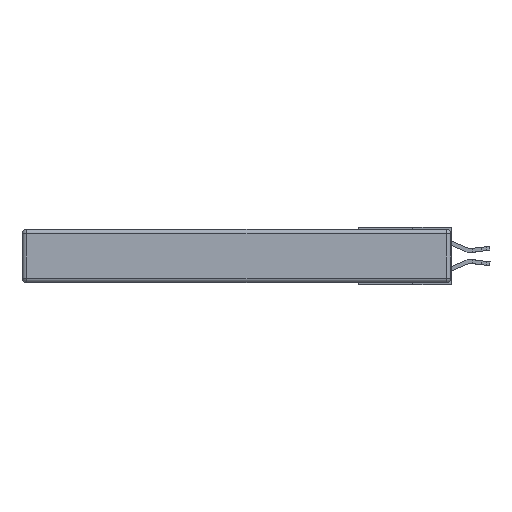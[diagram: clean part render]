
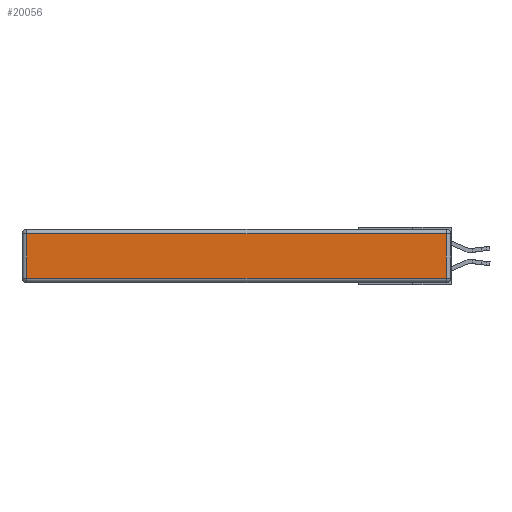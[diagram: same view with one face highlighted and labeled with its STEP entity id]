
A CAD part, left-side view. The second image highlights one B-rep face of the part: STEP entity #20056.
In plain terms, the highlighted planar face has unit normal (-1, 0, 0).
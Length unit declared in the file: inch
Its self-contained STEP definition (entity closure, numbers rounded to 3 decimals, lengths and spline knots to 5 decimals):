
#1045 = EDGE_CURVE ( 'NONE', #5660, #12351, #10678, .T. ) ;
#1574 = CARTESIAN_POINT ( 'NONE',  ( 0., 0., -0.313 ) ) ;
#1602 = CARTESIAN_POINT ( 'NONE',  ( 0., 0.03, -0.343 ) ) ;
#1655 = LINE ( 'NONE', #4994, #6934 ) ;
#3012 = LINE ( 'NONE', #17792, #17343 ) ;
#3937 = VERTEX_POINT ( 'NONE', #11427 ) ;
#4224 = VERTEX_POINT ( 'NONE', #5773 ) ;
#4994 = CARTESIAN_POINT ( 'NONE',  ( 0., 2.75, -0.03 ) ) ;
#5660 = VERTEX_POINT ( 'NONE', #11692 ) ;
#5773 = CARTESIAN_POINT ( 'NONE',  ( 0., 2.72, -0.313 ) ) ;
#5986 = DIRECTION ( 'NONE',  ( -1., 0., 0. ) ) ;
#6555 = AXIS2_PLACEMENT_3D ( 'NONE', #17345, #5986, #9339 ) ;
#6934 = VECTOR ( 'NONE', #19272, 39.37008 ) ;
#7466 = EDGE_CURVE ( 'NONE', #3937, #4224, #3012, .T. ) ;
#7895 = CARTESIAN_POINT ( 'NONE',  ( 0., 0.03, -0.03 ) ) ;
#9339 = DIRECTION ( 'NONE',  ( 0., 0., 1. ) ) ;
#9712 = ORIENTED_EDGE ( 'NONE', *, *, #1045, .T. ) ;
#9907 = VECTOR ( 'NONE', #17650, 39.37008 ) ;
#9934 = ORIENTED_EDGE ( 'NONE', *, *, #13434, .T. ) ;
#10027 = ORIENTED_EDGE ( 'NONE', *, *, #12484, .T. ) ;
#10678 = LINE ( 'NONE', #1602, #14408 ) ;
#11427 = CARTESIAN_POINT ( 'NONE',  ( 0., 2.72, -0.03 ) ) ;
#11692 = CARTESIAN_POINT ( 'NONE',  ( 0., 0.03, -0.313 ) ) ;
#12351 = VERTEX_POINT ( 'NONE', #7895 ) ;
#12484 = EDGE_CURVE ( 'NONE', #12351, #3937, #1655, .T. ) ;
#12853 = DIRECTION ( 'NONE',  ( 0., 0., 1. ) ) ;
#13434 = EDGE_CURVE ( 'NONE', #4224, #5660, #14176, .T. ) ;
#14115 = PLANE ( 'NONE',  #6555 ) ;
#14167 = EDGE_LOOP ( 'NONE', ( #9934, #9712, #10027, #20603 ) ) ;
#14176 = LINE ( 'NONE', #1574, #9907 ) ;
#14408 = VECTOR ( 'NONE', #12853, 39.37008 ) ;
#17343 = VECTOR ( 'NONE', #17989, 39.37008 ) ;
#17345 = CARTESIAN_POINT ( 'NONE',  ( 0., 0., -0.343 ) ) ;
#17650 = DIRECTION ( 'NONE',  ( 0., -1., 0. ) ) ;
#17792 = CARTESIAN_POINT ( 'NONE',  ( 0., 2.72, -0.343 ) ) ;
#17989 = DIRECTION ( 'NONE',  ( 0., 0., -1. ) ) ;
#18054 = FACE_OUTER_BOUND ( 'NONE', #14167, .T. ) ;
#19272 = DIRECTION ( 'NONE',  ( 0., 1., 0. ) ) ;
#20056 = ADVANCED_FACE ( 'NONE', ( #18054 ), #14115, .T. ) ;
#20603 = ORIENTED_EDGE ( 'NONE', *, *, #7466, .T. ) ;
